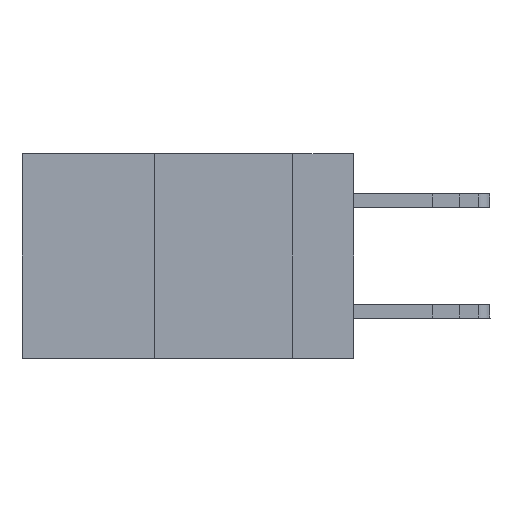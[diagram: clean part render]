
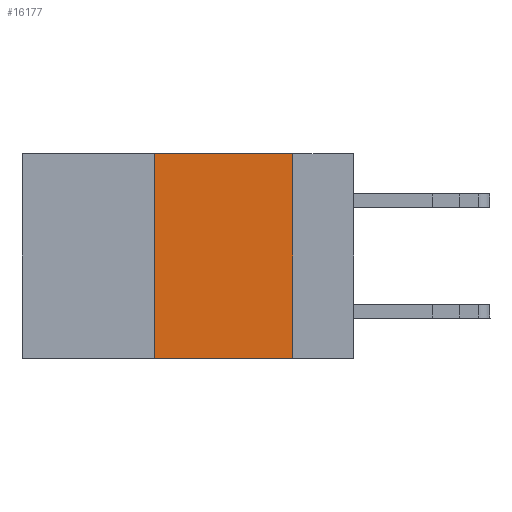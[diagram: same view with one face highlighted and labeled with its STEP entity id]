
A CAD part, left-side view. The second image highlights one B-rep face of the part: STEP entity #16177.
In plain terms, the highlighted planar face has unit normal (-1, 0, 0).
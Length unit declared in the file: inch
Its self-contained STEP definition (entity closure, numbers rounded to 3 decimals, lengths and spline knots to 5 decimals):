
#1522 = DIRECTION ( 'NONE',  ( 0., 0., -1. ) ) ;
#4271 = FACE_OUTER_BOUND ( 'NONE', #29194, .T. ) ;
#5248 = EDGE_CURVE ( 'NONE', #7762, #23935, #17298, .T. ) ;
#5352 = DIRECTION ( 'NONE',  ( 0., 0., 1. ) ) ;
#5364 = VECTOR ( 'NONE', #10549, 39.37008 ) ;
#5584 = CARTESIAN_POINT ( 'NONE',  ( 0., 0.36, -0.37 ) ) ;
#7502 = LINE ( 'NONE', #14227, #30104 ) ;
#7648 = DIRECTION ( 'NONE',  ( 0., -1., 0. ) ) ;
#7762 = VERTEX_POINT ( 'NONE', #5584 ) ;
#8125 = CARTESIAN_POINT ( 'NONE',  ( 0., 0.6, -0.37 ) ) ;
#9108 = CARTESIAN_POINT ( 'NONE',  ( 0., 0.11, 0. ) ) ;
#9880 = AXIS2_PLACEMENT_3D ( 'NONE', #18033, #24929, #1522 ) ;
#10549 = DIRECTION ( 'NONE',  ( 0., 0., -1. ) ) ;
#11297 = PLANE ( 'NONE',  #9880 ) ;
#13445 = LINE ( 'NONE', #29655, #5364 ) ;
#13665 = CARTESIAN_POINT ( 'NONE',  ( 0., 0.11, -0.37 ) ) ;
#13675 = ORIENTED_EDGE ( 'NONE', *, *, #5248, .T. ) ;
#14227 = CARTESIAN_POINT ( 'NONE',  ( 0., 0.36, 0. ) ) ;
#14688 = ORIENTED_EDGE ( 'NONE', *, *, #14803, .F. ) ;
#14803 = EDGE_CURVE ( 'NONE', #19080, #27295, #19270, .T. ) ;
#14920 = ORIENTED_EDGE ( 'NONE', *, *, #23232, .F. ) ;
#16177 = ADVANCED_FACE ( 'NONE', ( #4271 ), #11297, .F. ) ;
#16719 = ORIENTED_EDGE ( 'NONE', *, *, #28642, .F. ) ;
#17298 = LINE ( 'NONE', #8125, #18988 ) ;
#18033 = CARTESIAN_POINT ( 'NONE',  ( 0., 0.6, 0. ) ) ;
#18988 = VECTOR ( 'NONE', #26777, 39.37008 ) ;
#19080 = VERTEX_POINT ( 'NONE', #26970 ) ;
#19270 = LINE ( 'NONE', #29205, #25577 ) ;
#23232 = EDGE_CURVE ( 'NONE', #7762, #19080, #7502, .T. ) ;
#23935 = VERTEX_POINT ( 'NONE', #13665 ) ;
#24929 = DIRECTION ( 'NONE',  ( 1., 0., 0. ) ) ;
#25577 = VECTOR ( 'NONE', #7648, 39.37008 ) ;
#26777 = DIRECTION ( 'NONE',  ( 0., -1., 0. ) ) ;
#26970 = CARTESIAN_POINT ( 'NONE',  ( 0., 0.36, 0. ) ) ;
#27295 = VERTEX_POINT ( 'NONE', #9108 ) ;
#28642 = EDGE_CURVE ( 'NONE', #27295, #23935, #13445, .T. ) ;
#29194 = EDGE_LOOP ( 'NONE', ( #16719, #14688, #14920, #13675 ) ) ;
#29205 = CARTESIAN_POINT ( 'NONE',  ( 0., 0.6, 0. ) ) ;
#29655 = CARTESIAN_POINT ( 'NONE',  ( 0., 0.11, 0. ) ) ;
#30104 = VECTOR ( 'NONE', #5352, 39.37008 ) ;
